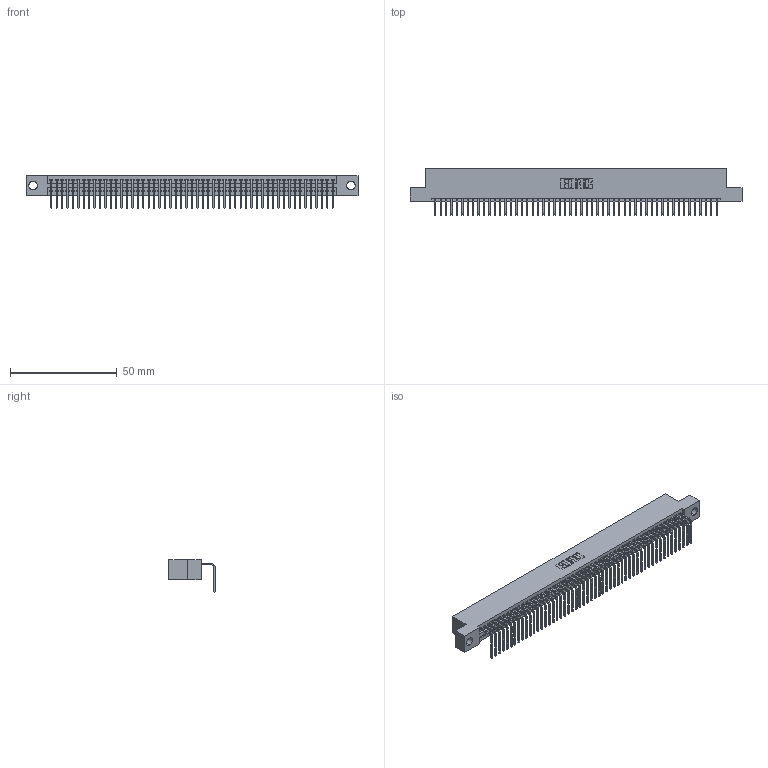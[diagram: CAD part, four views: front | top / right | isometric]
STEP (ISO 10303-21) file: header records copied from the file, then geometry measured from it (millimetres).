
FILE_DESCRIPTION (( 'STEP AP203' ), '1' );
FILE_NAME ('395-053-558-104.STEP', '2021-06-11T19:21:34', ( '' ), ( '' ), 'SwSTEP 2.0', 'SolidWorks 2020', '' );
FILE_SCHEMA (( 'CONFIG_CONTROL_DESIGN' ));
Length unit declared in the file: inch
Products named in the file (3): 345-292-001_558 Tail - 2; 345 Part_Flush Mounting Lugs - 0.156 Dia-TI; 395-053-558-104
Assembly tree (54 placements, depth 2):
  395-053-558-104
    345 Part_Flush Mounting Lugs - 0.156 Dia-TI
    345-292-001_558 Tail - 2  x53
Bounding box: 155.83 x 21.83 x 15.37 mm (x, y, z)
Volume: 14961.5 mm3; surface area: 20912.1 mm2
Topology: 54 solids, 54 shells, 3320 faces, 10023 edges, 6610 vertices
Faces by surface type: plane 2320, cylinder 1000
Entity records: 38911 total; most frequent: CARTESIAN_POINT 6749, ORIENTED_EDGE 6734, DIRECTION 5877, EDGE_CURVE 3367, LINE 3023, VECTOR 3023, VERTEX_POINT 2242, AXIS2_PLACEMENT_3D 1427
